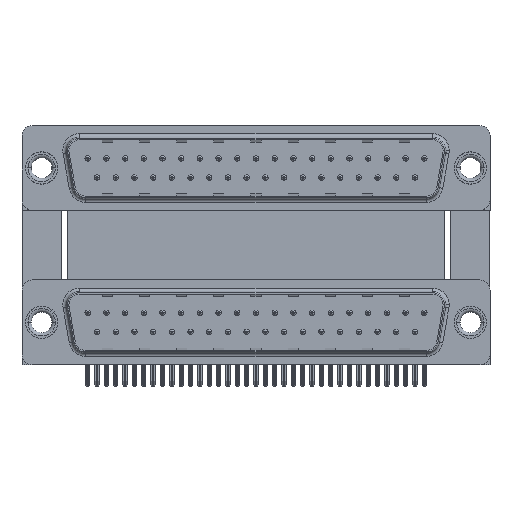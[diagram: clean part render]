
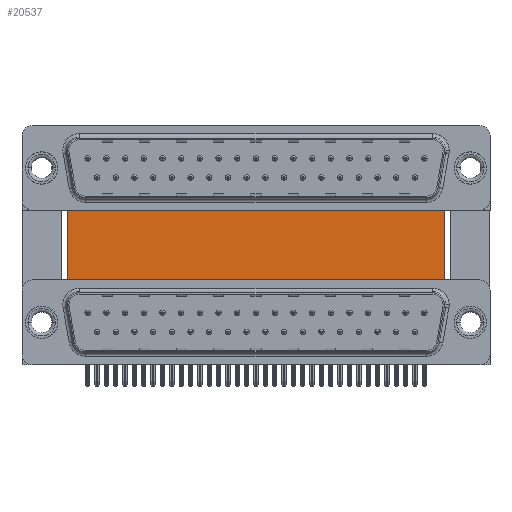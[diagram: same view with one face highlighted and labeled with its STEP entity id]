
A CAD part, top view. The second image highlights one B-rep face of the part: STEP entity #20537.
In plain terms, the highlighted planar face has unit normal (0, 0, 1).
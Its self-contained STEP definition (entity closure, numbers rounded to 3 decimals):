
#2885 = ORIENTED_EDGE ( 'NONE', *, *, #22598, .T. ) ;
#7147 = CARTESIAN_POINT ( 'NONE',  ( 3.79, 16.585, -12. ) ) ;
#9351 = LINE ( 'NONE', #20358, #18925 ) ;
#11498 = ORIENTED_EDGE ( 'NONE', *, *, #33416, .T. ) ;
#13279 = VECTOR ( 'NONE', #29028, 1000. ) ;
#14542 = VECTOR ( 'NONE', #38699, 1000. ) ;
#15467 = DIRECTION ( 'NONE',  ( 1., 0., 0. ) ) ;
#16149 = EDGE_CURVE ( 'NONE', #30656, #19283, #9351, .T. ) ;
#17314 = CARTESIAN_POINT ( 'NONE',  ( 59.71, -3.735, -12. ) ) ;
#18925 = VECTOR ( 'NONE', #20841, 1000. ) ;
#19283 = VERTEX_POINT ( 'NONE', #17314 ) ;
#19372 = LINE ( 'NONE', #41641, #14542 ) ;
#20358 = CARTESIAN_POINT ( 'NONE',  ( 59.71, 16.585, -12. ) ) ;
#20537 = ADVANCED_FACE ( 'NONE', ( #29664 ), #25736, .F. ) ;
#20841 = DIRECTION ( 'NONE',  ( 0., -1., 0. ) ) ;
#22071 = DIRECTION ( 'NONE',  ( 0., 0., -1. ) ) ;
#22598 = EDGE_CURVE ( 'NONE', #33467, #44290, #19372, .T. ) ;
#24583 = AXIS2_PLACEMENT_3D ( 'NONE', #7147, #22071, #37020 ) ;
#25736 = PLANE ( 'NONE',  #24583 ) ;
#26327 = CARTESIAN_POINT ( 'NONE',  ( 3.79, -3.735, -12. ) ) ;
#28398 = ORIENTED_EDGE ( 'NONE', *, *, #44432, .F. ) ;
#29028 = DIRECTION ( 'NONE',  ( 1., 0., 0. ) ) ;
#29643 = EDGE_LOOP ( 'NONE', ( #11498, #42388, #28398, #2885 ) ) ;
#29664 = FACE_OUTER_BOUND ( 'NONE', #29643, .T. ) ;
#30656 = VERTEX_POINT ( 'NONE', #35964 ) ;
#31083 = VECTOR ( 'NONE', #15467, 1000. ) ;
#32718 = LINE ( 'NONE', #26327, #13279 ) ;
#33416 = EDGE_CURVE ( 'NONE', #44290, #19283, #32718, .T. ) ;
#33441 = CARTESIAN_POINT ( 'NONE',  ( 3.79, 16.585, -12. ) ) ;
#33467 = VERTEX_POINT ( 'NONE', #33441 ) ;
#35964 = CARTESIAN_POINT ( 'NONE',  ( 59.71, 16.585, -12. ) ) ;
#37020 = DIRECTION ( 'NONE',  ( -1., 0., 0. ) ) ;
#37744 = CARTESIAN_POINT ( 'NONE',  ( 3.79, 16.585, -12. ) ) ;
#38699 = DIRECTION ( 'NONE',  ( 0., -1., 0. ) ) ;
#41641 = CARTESIAN_POINT ( 'NONE',  ( 3.79, 16.585, -12. ) ) ;
#42388 = ORIENTED_EDGE ( 'NONE', *, *, #16149, .F. ) ;
#44290 = VERTEX_POINT ( 'NONE', #47574 ) ;
#44432 = EDGE_CURVE ( 'NONE', #33467, #30656, #45348, .T. ) ;
#45348 = LINE ( 'NONE', #37744, #31083 ) ;
#47574 = CARTESIAN_POINT ( 'NONE',  ( 3.79, -3.735, -12. ) ) ;
